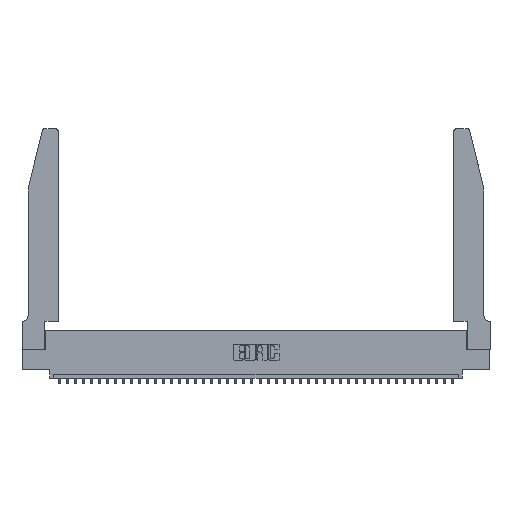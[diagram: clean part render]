
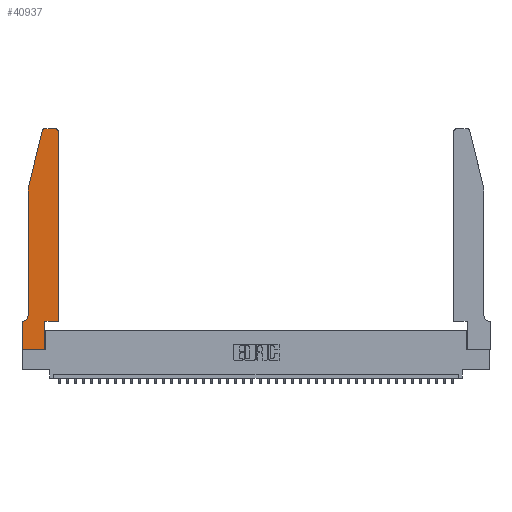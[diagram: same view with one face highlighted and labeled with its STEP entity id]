
A CAD part, top view. The second image highlights one B-rep face of the part: STEP entity #40937.
In plain terms, the highlighted planar face has unit normal (0, 0, 1).
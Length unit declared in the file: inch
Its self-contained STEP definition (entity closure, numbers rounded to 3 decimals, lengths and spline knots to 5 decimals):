
#70 = ORIENTED_EDGE ( 'NONE', *, *, #34965, .T. ) ;
#245 = CARTESIAN_POINT ( 'NONE',  ( 0.284, 2.72, 0.37 ) ) ;
#716 = DIRECTION ( 'NONE',  ( 1., 0., 0. ) ) ;
#1367 = AXIS2_PLACEMENT_3D ( 'NONE', #34318, #2700, #5506 ) ;
#2700 = DIRECTION ( 'NONE',  ( 0., 0., -1. ) ) ;
#2852 = LINE ( 'NONE', #11486, #5383 ) ;
#2900 = CARTESIAN_POINT ( 'NONE',  ( 0., 0.35, 0.37 ) ) ;
#4273 = LINE ( 'NONE', #24917, #38863 ) ;
#4508 = DIRECTION ( 'NONE',  ( 0., -1., 0. ) ) ;
#4700 = VERTEX_POINT ( 'NONE', #9288 ) ;
#4908 = VERTEX_POINT ( 'NONE', #18591 ) ;
#5077 = CARTESIAN_POINT ( 'NONE',  ( 0.2605, 2.75, 0.37 ) ) ;
#5383 = VECTOR ( 'NONE', #40377, 39.37008 ) ;
#5506 = DIRECTION ( 'NONE',  ( -1., 0., 0. ) ) ;
#7181 = EDGE_CURVE ( 'NONE', #8198, #14017, #4273, .T. ) ;
#8198 = VERTEX_POINT ( 'NONE', #38111 ) ;
#8266 = EDGE_CURVE ( 'NONE', #37970, #26491, #13198, .T. ) ;
#8706 = CARTESIAN_POINT ( 'NONE',  ( 0.0755, 0.35, 0.37 ) ) ;
#9288 = CARTESIAN_POINT ( 'NONE',  ( 0., 0.35, 0.37 ) ) ;
#9364 = VECTOR ( 'NONE', #11952, 39.37008 ) ;
#9833 = EDGE_CURVE ( 'NONE', #34460, #39883, #30233, .T. ) ;
#11486 = CARTESIAN_POINT ( 'NONE',  ( 0.0755, 2., 0.37 ) ) ;
#11604 = VECTOR ( 'NONE', #20637, 39.37008 ) ;
#11720 = AXIS2_PLACEMENT_3D ( 'NONE', #23173, #30032, #716 ) ;
#11952 = DIRECTION ( 'NONE',  ( 1., 0., 0. ) ) ;
#12063 = DIRECTION ( 'NONE',  ( -1., 0., 0. ) ) ;
#12268 = DIRECTION ( 'NONE',  ( 0., 1., 0. ) ) ;
#12375 = CARTESIAN_POINT ( 'NONE',  ( 0.4505, 0.35, 0.37 ) ) ;
#12656 = CIRCLE ( 'NONE', #1367, 0.07 ) ;
#13130 = ORIENTED_EDGE ( 'NONE', *, *, #41513, .T. ) ;
#13185 = VECTOR ( 'NONE', #38200, 39.37008 ) ;
#13198 = LINE ( 'NONE', #5077, #30744 ) ;
#13600 = CARTESIAN_POINT ( 'NONE',  ( 0.284, 2.75, 0.37 ) ) ;
#13845 = LINE ( 'NONE', #38016, #9364 ) ;
#14017 = VERTEX_POINT ( 'NONE', #29841 ) ;
#14221 = EDGE_LOOP ( 'NONE', ( #30309, #19575, #27249, #25452, #20966, #37173, #15912, #15920, #14831, #13130, #70, #18720 ) ) ;
#14690 = EDGE_CURVE ( 'NONE', #25637, #4700, #25353, .T. ) ;
#14831 = ORIENTED_EDGE ( 'NONE', *, *, #22668, .T. ) ;
#15347 = VERTEX_POINT ( 'NONE', #36509 ) ;
#15789 = DIRECTION ( 'NONE',  ( 1., 0., 0. ) ) ;
#15800 = CARTESIAN_POINT ( 'NONE',  ( 0., 0., 0.37 ) ) ;
#15912 = ORIENTED_EDGE ( 'NONE', *, *, #32431, .T. ) ;
#15920 = ORIENTED_EDGE ( 'NONE', *, *, #9833, .T. ) ;
#18084 = CARTESIAN_POINT ( 'NONE',  ( 0.0055, 0.35, 0.37 ) ) ;
#18490 = EDGE_CURVE ( 'NONE', #14017, #25637, #12656, .T. ) ;
#18591 = CARTESIAN_POINT ( 'NONE',  ( 0.2865, 0.35, 0.37 ) ) ;
#18720 = ORIENTED_EDGE ( 'NONE', *, *, #31970, .T. ) ;
#19201 = DIRECTION ( 'NONE',  ( 0., 0., 1. ) ) ;
#19575 = ORIENTED_EDGE ( 'NONE', *, *, #31234, .T. ) ;
#20637 = DIRECTION ( 'NONE',  ( 0., 1., 0. ) ) ;
#20966 = ORIENTED_EDGE ( 'NONE', *, *, #18490, .T. ) ;
#21905 = VECTOR ( 'NONE', #40949, 39.37008 ) ;
#22089 = PLANE ( 'NONE',  #28061 ) ;
#22382 = CARTESIAN_POINT ( 'NONE',  ( 0.4205, 2.75, 0.37 ) ) ;
#22668 = EDGE_CURVE ( 'NONE', #39883, #4908, #37156, .T. ) ;
#23173 = CARTESIAN_POINT ( 'NONE',  ( 0.4205, 2.72, 0.37 ) ) ;
#23456 = CARTESIAN_POINT ( 'NONE',  ( 0.4505, 2.72, 0.37 ) ) ;
#24658 = CIRCLE ( 'NONE', #11720, 0.03 ) ;
#24721 = CARTESIAN_POINT ( 'NONE',  ( 0.4505, 0.35, 0.37 ) ) ;
#24917 = CARTESIAN_POINT ( 'NONE',  ( 0.0755, 2., 0.37 ) ) ;
#25285 = DIRECTION ( 'NONE',  ( 0., 0., 1. ) ) ;
#25353 = LINE ( 'NONE', #8706, #21905 ) ;
#25452 = ORIENTED_EDGE ( 'NONE', *, *, #7181, .T. ) ;
#25468 = DIRECTION ( 'NONE',  ( 0., -1., 0. ) ) ;
#25629 = DIRECTION ( 'NONE',  ( 1., 0., 0. ) ) ;
#25637 = VERTEX_POINT ( 'NONE', #18084 ) ;
#26491 = VERTEX_POINT ( 'NONE', #13600 ) ;
#27249 = ORIENTED_EDGE ( 'NONE', *, *, #37333, .T. ) ;
#27930 = FACE_OUTER_BOUND ( 'NONE', #14221, .T. ) ;
#28061 = AXIS2_PLACEMENT_3D ( 'NONE', #2900, #25285, #15789 ) ;
#29109 = VERTEX_POINT ( 'NONE', #23456 ) ;
#29841 = CARTESIAN_POINT ( 'NONE',  ( 0.0755, 0.42, 0.37 ) ) ;
#30032 = DIRECTION ( 'NONE',  ( 0., 0., 1. ) ) ;
#30233 = LINE ( 'NONE', #15800, #13185 ) ;
#30309 = ORIENTED_EDGE ( 'NONE', *, *, #8266, .T. ) ;
#30431 = CARTESIAN_POINT ( 'NONE',  ( 0.2865, 0.35, 0.37 ) ) ;
#30744 = VECTOR ( 'NONE', #12063, 39.37008 ) ;
#31234 = EDGE_CURVE ( 'NONE', #26491, #15347, #35233, .T. ) ;
#31970 = EDGE_CURVE ( 'NONE', #29109, #37970, #24658, .T. ) ;
#32431 = EDGE_CURVE ( 'NONE', #4700, #34460, #35125, .T. ) ;
#34318 = CARTESIAN_POINT ( 'NONE',  ( 0.0055, 0.42, 0.37 ) ) ;
#34460 = VERTEX_POINT ( 'NONE', #35227 ) ;
#34965 = EDGE_CURVE ( 'NONE', #41467, #29109, #39278, .T. ) ;
#35125 = LINE ( 'NONE', #36562, #41198 ) ;
#35227 = CARTESIAN_POINT ( 'NONE',  ( 0., 0., 0.37 ) ) ;
#35233 = CIRCLE ( 'NONE', #35502, 0.03 ) ;
#35502 = AXIS2_PLACEMENT_3D ( 'NONE', #245, #19201, #25629 ) ;
#36509 = CARTESIAN_POINT ( 'NONE',  ( 0.25487, 2.72718, 0.37 ) ) ;
#36562 = CARTESIAN_POINT ( 'NONE',  ( 0., 0., 0.37 ) ) ;
#36818 = CARTESIAN_POINT ( 'NONE',  ( 0.2865, 0., 0.37 ) ) ;
#37156 = LINE ( 'NONE', #30431, #11604 ) ;
#37173 = ORIENTED_EDGE ( 'NONE', *, *, #14690, .T. ) ;
#37333 = EDGE_CURVE ( 'NONE', #15347, #8198, #2852, .T. ) ;
#37970 = VERTEX_POINT ( 'NONE', #22382 ) ;
#38016 = CARTESIAN_POINT ( 'NONE',  ( 0.4505, 0.35, 0.37 ) ) ;
#38111 = CARTESIAN_POINT ( 'NONE',  ( 0.0755, 2., 0.37 ) ) ;
#38200 = DIRECTION ( 'NONE',  ( 1., 0., 0. ) ) ;
#38863 = VECTOR ( 'NONE', #25468, 39.37008 ) ;
#39278 = LINE ( 'NONE', #24721, #40270 ) ;
#39883 = VERTEX_POINT ( 'NONE', #36818 ) ;
#40270 = VECTOR ( 'NONE', #12268, 39.37008 ) ;
#40377 = DIRECTION ( 'NONE',  ( -0.239, -0.971, 0. ) ) ;
#40937 = ADVANCED_FACE ( 'NONE', ( #27930 ), #22089, .T. ) ;
#40949 = DIRECTION ( 'NONE',  ( -1., 0., 0. ) ) ;
#41198 = VECTOR ( 'NONE', #4508, 39.37008 ) ;
#41467 = VERTEX_POINT ( 'NONE', #12375 ) ;
#41513 = EDGE_CURVE ( 'NONE', #4908, #41467, #13845, .T. ) ;
